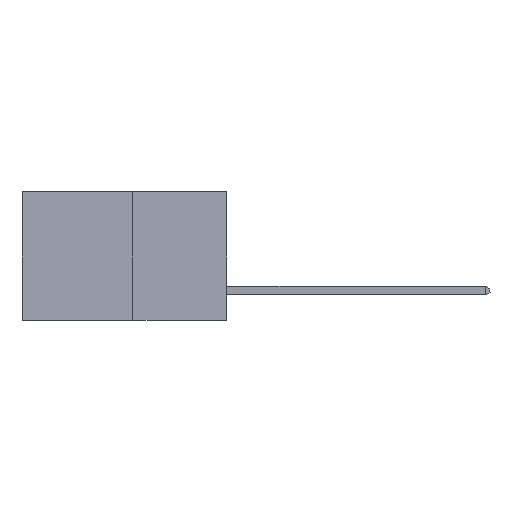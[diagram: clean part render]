
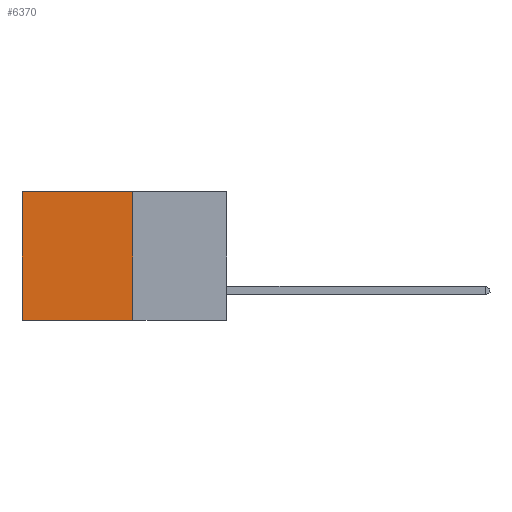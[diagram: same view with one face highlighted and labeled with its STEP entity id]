
A CAD part, left-side view. The second image highlights one B-rep face of the part: STEP entity #6370.
In plain terms, the highlighted planar face has unit normal (-1, 0, 0).
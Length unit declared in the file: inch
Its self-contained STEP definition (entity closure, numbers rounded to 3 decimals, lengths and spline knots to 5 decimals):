
#975 = VERTEX_POINT ( 'NONE', #8032 ) ;
#1007 = CARTESIAN_POINT ( 'NONE',  ( 0.277, 0.27, -0.37 ) ) ;
#1814 = VECTOR ( 'NONE', #18017, 39.37008 ) ;
#2110 = EDGE_LOOP ( 'NONE', ( #9396, #8183, #15026, #7321 ) ) ;
#2404 = PLANE ( 'NONE',  #15361 ) ;
#4359 = EDGE_CURVE ( 'NONE', #8138, #6751, #9195, .T. ) ;
#5260 = DIRECTION ( 'NONE',  ( 0., 0., -1. ) ) ;
#6370 = ADVANCED_FACE ( 'NONE', ( #7554 ), #2404, .F. ) ;
#6751 = VERTEX_POINT ( 'NONE', #10264 ) ;
#6915 = CARTESIAN_POINT ( 'NONE',  ( 0.277, 0.27, -0.37 ) ) ;
#7020 = VECTOR ( 'NONE', #7309, 39.37008 ) ;
#7309 = DIRECTION ( 'NONE',  ( 0., 1., 0. ) ) ;
#7321 = ORIENTED_EDGE ( 'NONE', *, *, #4359, .T. ) ;
#7554 = FACE_OUTER_BOUND ( 'NONE', #2110, .T. ) ;
#8032 = CARTESIAN_POINT ( 'NONE',  ( 0.277, 0.59, -0.37 ) ) ;
#8102 = CARTESIAN_POINT ( 'NONE',  ( 0.277, 0.59, -0.37 ) ) ;
#8138 = VERTEX_POINT ( 'NONE', #16261 ) ;
#8183 = ORIENTED_EDGE ( 'NONE', *, *, #9196, .F. ) ;
#8467 = LINE ( 'NONE', #8102, #1814 ) ;
#9195 = LINE ( 'NONE', #16565, #12522 ) ;
#9196 = EDGE_CURVE ( 'NONE', #16464, #975, #11218, .T. ) ;
#9396 = ORIENTED_EDGE ( 'NONE', *, *, #11468, .T. ) ;
#9961 = DIRECTION ( 'NONE',  ( 0., 0., -1. ) ) ;
#10264 = CARTESIAN_POINT ( 'NONE',  ( 0.277, 0.59, 0. ) ) ;
#10355 = EDGE_CURVE ( 'NONE', #8138, #16464, #13397, .T. ) ;
#11218 = LINE ( 'NONE', #14371, #7020 ) ;
#11468 = EDGE_CURVE ( 'NONE', #6751, #975, #8467, .T. ) ;
#12522 = VECTOR ( 'NONE', #17986, 39.37008 ) ;
#13397 = LINE ( 'NONE', #14278, #16724 ) ;
#13765 = DIRECTION ( 'NONE',  ( 1., 0., 0. ) ) ;
#14278 = CARTESIAN_POINT ( 'NONE',  ( 0.277, 0.27, -0.37 ) ) ;
#14371 = CARTESIAN_POINT ( 'NONE',  ( 0.277, 0.27, -0.37 ) ) ;
#15026 = ORIENTED_EDGE ( 'NONE', *, *, #10355, .F. ) ;
#15361 = AXIS2_PLACEMENT_3D ( 'NONE', #1007, #13765, #5260 ) ;
#16261 = CARTESIAN_POINT ( 'NONE',  ( 0.277, 0.27, 0. ) ) ;
#16464 = VERTEX_POINT ( 'NONE', #6915 ) ;
#16565 = CARTESIAN_POINT ( 'NONE',  ( 0.277, 0.27, 0. ) ) ;
#16724 = VECTOR ( 'NONE', #9961, 39.37008 ) ;
#17986 = DIRECTION ( 'NONE',  ( 0., 1., 0. ) ) ;
#18017 = DIRECTION ( 'NONE',  ( 0., 0., -1. ) ) ;
